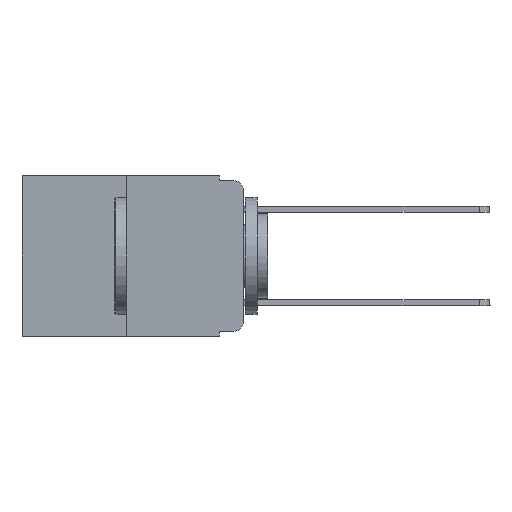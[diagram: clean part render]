
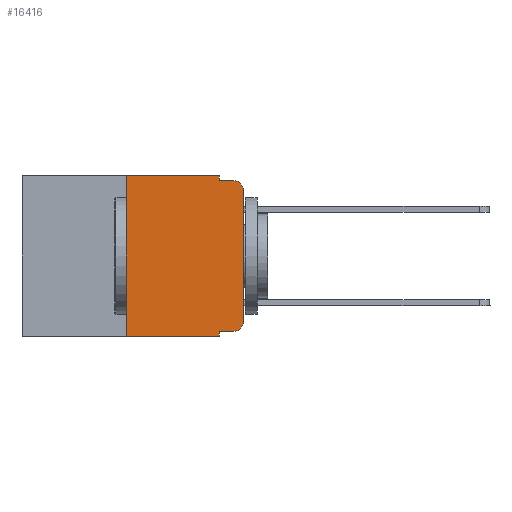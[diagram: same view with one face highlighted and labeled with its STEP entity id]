
A CAD part, left-side view. The second image highlights one B-rep face of the part: STEP entity #16416.
In plain terms, the highlighted planar face has unit normal (-1, 0, 0).
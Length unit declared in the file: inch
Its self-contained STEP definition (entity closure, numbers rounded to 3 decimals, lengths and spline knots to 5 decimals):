
#88 = LINE ( 'NONE', #13927, #17941 ) ;
#564 = CARTESIAN_POINT ( 'NONE',  ( 0., 0.051, 0. ) ) ;
#576 = VERTEX_POINT ( 'NONE', #9879 ) ;
#978 = VECTOR ( 'NONE', #11953, 39.37008 ) ;
#1261 = EDGE_CURVE ( 'NONE', #576, #3886, #18816, .T. ) ;
#1832 = PLANE ( 'NONE',  #7389 ) ;
#2039 = LINE ( 'NONE', #2696, #21301 ) ;
#2505 = VERTEX_POINT ( 'NONE', #3415 ) ;
#2696 = CARTESIAN_POINT ( 'NONE',  ( 0., 0.051, -0.01 ) ) ;
#3043 = CIRCLE ( 'NONE', #21171, 0.02 ) ;
#3248 = EDGE_CURVE ( 'NONE', #576, #5186, #6739, .T. ) ;
#3415 = CARTESIAN_POINT ( 'NONE',  ( 0., 0.051, 0. ) ) ;
#3515 = DIRECTION ( 'NONE',  ( 0., -1., 0. ) ) ;
#3645 = LINE ( 'NONE', #19999, #978 ) ;
#3886 = VERTEX_POINT ( 'NONE', #11982 ) ;
#4225 = CARTESIAN_POINT ( 'NONE',  ( 0., 0.02, -0.01 ) ) ;
#4632 = CARTESIAN_POINT ( 'NONE',  ( 0., 0.02, -0.313 ) ) ;
#4973 = CARTESIAN_POINT ( 'NONE',  ( 0., 0.25, -0.343 ) ) ;
#5186 = VERTEX_POINT ( 'NONE', #23532 ) ;
#5424 = DIRECTION ( 'NONE',  ( 0., 0., -1. ) ) ;
#5775 = DIRECTION ( 'NONE',  ( 0., 0., -1. ) ) ;
#5839 = VERTEX_POINT ( 'NONE', #10352 ) ;
#5947 = CARTESIAN_POINT ( 'NONE',  ( 0., 0.02, -0.03 ) ) ;
#5995 = DIRECTION ( 'NONE',  ( 0., 0., 1. ) ) ;
#6739 = LINE ( 'NONE', #564, #7379 ) ;
#6859 = VERTEX_POINT ( 'NONE', #22420 ) ;
#7006 = DIRECTION ( 'NONE',  ( 0., 0., -1. ) ) ;
#7204 = ORIENTED_EDGE ( 'NONE', *, *, #11896, .T. ) ;
#7379 = VECTOR ( 'NONE', #7006, 39.37008 ) ;
#7389 = AXIS2_PLACEMENT_3D ( 'NONE', #24298, #7898, #5775 ) ;
#7541 = DIRECTION ( 'NONE',  ( -1., 0., 0. ) ) ;
#7576 = ORIENTED_EDGE ( 'NONE', *, *, #16742, .F. ) ;
#7662 = VECTOR ( 'NONE', #5995, 39.37008 ) ;
#7898 = DIRECTION ( 'NONE',  ( 1., 0., 0. ) ) ;
#8269 = DIRECTION ( 'NONE',  ( 0., -1., 0. ) ) ;
#8339 = DIRECTION ( 'NONE',  ( 0., 0., -1. ) ) ;
#9220 = EDGE_CURVE ( 'NONE', #3886, #10213, #3043, .T. ) ;
#9550 = VECTOR ( 'NONE', #3515, 39.37008 ) ;
#9830 = LINE ( 'NONE', #23759, #21403 ) ;
#9879 = CARTESIAN_POINT ( 'NONE',  ( 0., 0.051, -0.333 ) ) ;
#10213 = VERTEX_POINT ( 'NONE', #19097 ) ;
#10352 = CARTESIAN_POINT ( 'NONE',  ( 0., 0., -0.03 ) ) ;
#10744 = VERTEX_POINT ( 'NONE', #18639 ) ;
#11896 = EDGE_CURVE ( 'NONE', #19105, #5186, #3645, .T. ) ;
#11953 = DIRECTION ( 'NONE',  ( 0., -1., 0. ) ) ;
#11982 = CARTESIAN_POINT ( 'NONE',  ( 0., 0.02, -0.333 ) ) ;
#12095 = ORIENTED_EDGE ( 'NONE', *, *, #17693, .T. ) ;
#13471 = VECTOR ( 'NONE', #8269, 39.37008 ) ;
#13527 = CARTESIAN_POINT ( 'NONE',  ( 0., 0.473, 0. ) ) ;
#13927 = CARTESIAN_POINT ( 'NONE',  ( 0., 0.051, 0. ) ) ;
#13980 = ORIENTED_EDGE ( 'NONE', *, *, #15656, .F. ) ;
#14141 = CARTESIAN_POINT ( 'NONE',  ( 0., 0., 0. ) ) ;
#15085 = EDGE_CURVE ( 'NONE', #2505, #10744, #88, .T. ) ;
#15656 = EDGE_CURVE ( 'NONE', #10744, #19680, #2039, .T. ) ;
#15663 = FACE_OUTER_BOUND ( 'NONE', #19445, .T. ) ;
#16416 = ADVANCED_FACE ( 'NONE', ( #15663 ), #1832, .F. ) ;
#16742 = EDGE_CURVE ( 'NONE', #6859, #2505, #16972, .T. ) ;
#16746 = ORIENTED_EDGE ( 'NONE', *, *, #3248, .F. ) ;
#16972 = LINE ( 'NONE', #13527, #9550 ) ;
#17693 = EDGE_CURVE ( 'NONE', #5839, #19680, #18785, .T. ) ;
#17881 = LINE ( 'NONE', #14141, #7662 ) ;
#17941 = VECTOR ( 'NONE', #25907, 39.37008 ) ;
#18218 = ORIENTED_EDGE ( 'NONE', *, *, #1261, .T. ) ;
#18639 = CARTESIAN_POINT ( 'NONE',  ( 0., 0.051, -0.01 ) ) ;
#18785 = CIRCLE ( 'NONE', #21781, 0.02 ) ;
#18816 = LINE ( 'NONE', #22801, #13471 ) ;
#19097 = CARTESIAN_POINT ( 'NONE',  ( 0., 0., -0.313 ) ) ;
#19105 = VERTEX_POINT ( 'NONE', #4973 ) ;
#19169 = EDGE_CURVE ( 'NONE', #19105, #6859, #9830, .T. ) ;
#19445 = EDGE_LOOP ( 'NONE', ( #24674, #12095, #13980, #20998, #7576, #21993, #7204, #16746, #18218, #25334 ) ) ;
#19680 = VERTEX_POINT ( 'NONE', #4225 ) ;
#19999 = CARTESIAN_POINT ( 'NONE',  ( 0., 0.473, -0.343 ) ) ;
#20748 = DIRECTION ( 'NONE',  ( -1., 0., 0. ) ) ;
#20998 = ORIENTED_EDGE ( 'NONE', *, *, #15085, .F. ) ;
#21171 = AXIS2_PLACEMENT_3D ( 'NONE', #4632, #20748, #8339 ) ;
#21301 = VECTOR ( 'NONE', #22251, 39.37008 ) ;
#21403 = VECTOR ( 'NONE', #21880, 39.37008 ) ;
#21781 = AXIS2_PLACEMENT_3D ( 'NONE', #5947, #7541, #5424 ) ;
#21880 = DIRECTION ( 'NONE',  ( 0., 0., 1. ) ) ;
#21993 = ORIENTED_EDGE ( 'NONE', *, *, #19169, .F. ) ;
#22251 = DIRECTION ( 'NONE',  ( 0., -1., 0. ) ) ;
#22420 = CARTESIAN_POINT ( 'NONE',  ( 0., 0.25, 0. ) ) ;
#22801 = CARTESIAN_POINT ( 'NONE',  ( 0., 0.051, -0.333 ) ) ;
#23532 = CARTESIAN_POINT ( 'NONE',  ( 0., 0.051, -0.343 ) ) ;
#23759 = CARTESIAN_POINT ( 'NONE',  ( 0., 0.25, 0. ) ) ;
#24298 = CARTESIAN_POINT ( 'NONE',  ( 0., 0.473, 0. ) ) ;
#24674 = ORIENTED_EDGE ( 'NONE', *, *, #25064, .T. ) ;
#25064 = EDGE_CURVE ( 'NONE', #10213, #5839, #17881, .T. ) ;
#25334 = ORIENTED_EDGE ( 'NONE', *, *, #9220, .T. ) ;
#25907 = DIRECTION ( 'NONE',  ( 0., 0., -1. ) ) ;
